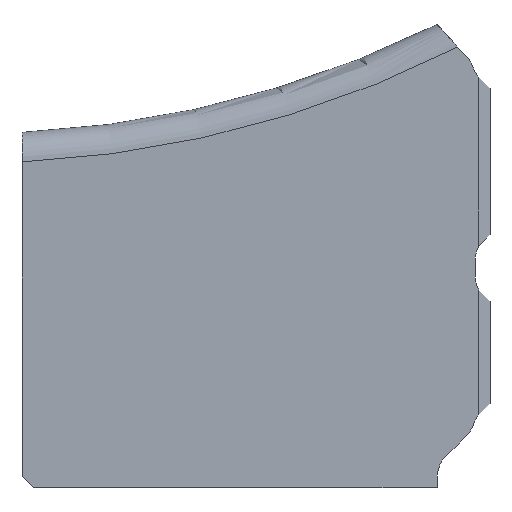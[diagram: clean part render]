
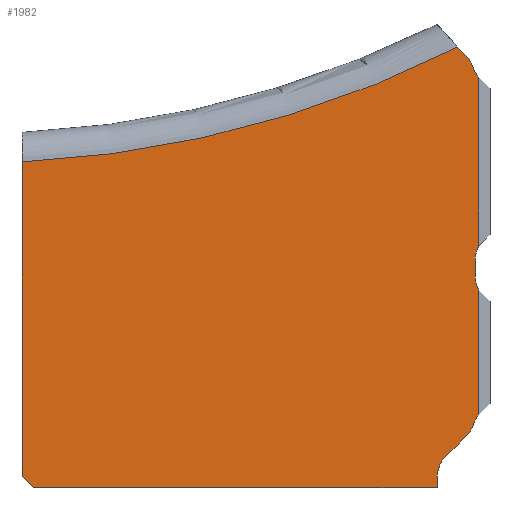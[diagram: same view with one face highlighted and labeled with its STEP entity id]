
A CAD part, front view. The second image highlights one B-rep face of the part: STEP entity #1982.
In plain terms, the highlighted planar face has unit normal (0, -1, 0).
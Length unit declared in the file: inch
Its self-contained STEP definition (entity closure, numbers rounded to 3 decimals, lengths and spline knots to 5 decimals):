
#145 = CIRCLE ( 'NONE', #2823, 0.3937 ) ;
#146 = CIRCLE ( 'NONE', #2832, 0.3937 ) ;
#149 = CIRCLE ( 'NONE', #2792, 0.3937 ) ;
#150 = CIRCLE ( 'NONE', #2861, 0.3937 ) ;
#164 = CIRCLE ( 'NONE', #2778, 14.52805 ) ;
#172 = CIRCLE ( 'NONE', #2789, 0.3937 ) ;
#173 = CIRCLE ( 'NONE', #2790, 0.3937 ) ;
#174 = CIRCLE ( 'NONE', #2833, 0.3937 ) ;
#375 = PLANE ( 'NONE',  #3064 ) ;
#376 = CARTESIAN_POINT ( 'NONE',  ( 0., 0., 0. ) ) ;
#379 = DIRECTION ( 'NONE',  ( 0., 1., 0. ) ) ;
#412 = DIRECTION ( 'NONE',  ( 0., 0., 1. ) ) ;
#1637 = CARTESIAN_POINT ( 'NONE',  ( 0., 0., 0. ) ) ;
#1642 = DIRECTION ( 'NONE',  ( 0., 0., -1. ) ) ;
#1646 = CARTESIAN_POINT ( 'NONE',  ( 5.66581, 0., 0.73541 ) ) ;
#1649 = DIRECTION ( 'NONE',  ( 0., -1., 0. ) ) ;
#1650 = LINE ( 'NONE', #1637, #2796 ) ;
#1663 = DIRECTION ( 'NONE',  ( 0., 1., 0. ) ) ;
#1670 = CARTESIAN_POINT ( 'NONE',  ( -0.70452, 0., 14.11678 ) ) ;
#1671 = DIRECTION ( 'NONE',  ( 0., 0., 1. ) ) ;
#1676 = LINE ( 'NONE', #1678, #2814 ) ;
#1677 = DIRECTION ( 'NONE',  ( 0.707, 0., 0.707 ) ) ;
#1678 = CARTESIAN_POINT ( 'NONE',  ( 5.00113, 0., -5.00113 ) ) ;
#1685 = DIRECTION ( 'NONE',  ( 0., 0., 1. ) ) ;
#1686 = CARTESIAN_POINT ( 'NONE',  ( 6.41166, 0., 0.9878 ) ) ;
#1687 = DIRECTION ( 'NONE',  ( 0., 0., 1. ) ) ;
#1688 = DIRECTION ( 'NONE',  ( 0., 1., 0. ) ) ;
#1690 = LINE ( 'NONE', #1691, #2801 ) ;
#1691 = CARTESIAN_POINT ( 'NONE',  ( 6.05951, 0., 0. ) ) ;
#1692 = DIRECTION ( 'NONE',  ( 0., 0., 1. ) ) ;
#1703 = LINE ( 'NONE', #1726, #2809 ) ;
#1711 = CARTESIAN_POINT ( 'NONE',  ( 6.10951, 0., 0. ) ) ;
#1718 = LINE ( 'NONE', #1711, #2817 ) ;
#1724 = DIRECTION ( 'NONE',  ( 0., 0., 1. ) ) ;
#1725 = DIRECTION ( 'NONE',  ( 0., 0., 1. ) ) ;
#1726 = CARTESIAN_POINT ( 'NONE',  ( 5.55226, 0., -4.75 ) ) ;
#1731 = DIRECTION ( 'NONE',  ( 0., 1., 0. ) ) ;
#1732 = CARTESIAN_POINT ( 'NONE',  ( 5.55226, 0., -4.75 ) ) ;
#1733 = DIRECTION ( 'NONE',  ( -1., 0., 0. ) ) ;
#1735 = LINE ( 'NONE', #1756, #2816 ) ;
#1739 = DIRECTION ( 'NONE',  ( 0.707, 0., -0.707 ) ) ;
#1741 = CARTESIAN_POINT ( 'NONE',  ( 6.45321, 0., -1.71415 ) ) ;
#1744 = LINE ( 'NONE', #1732, #2807 ) ;
#1753 = DIRECTION ( 'NONE',  ( 0., 0., 1. ) ) ;
#1756 = CARTESIAN_POINT ( 'NONE',  ( 0.15, 0., -4.75 ) ) ;
#1791 = LINE ( 'NONE', #1809, #2829 ) ;
#1792 = CARTESIAN_POINT ( 'NONE',  ( 6.10951, 0., 0. ) ) ;
#1800 = DIRECTION ( 'NONE',  ( -0.675, 0., 0.738 ) ) ;
#1802 = LINE ( 'NONE', #1792, #2831 ) ;
#1809 = CARTESIAN_POINT ( 'NONE',  ( 3.74048, 0., 3.42269 ) ) ;
#1818 = DIRECTION ( 'NONE',  ( 0., 0., 1. ) ) ;
#1854 = CARTESIAN_POINT ( 'NONE',  ( 6.41166, 0., -4.03208 ) ) ;
#1856 = DIRECTION ( 'NONE',  ( 0., 1., 0. ) ) ;
#1858 = CARTESIAN_POINT ( 'NONE',  ( 5.66581, 0., -3.77968 ) ) ;
#1859 = DIRECTION ( 'NONE',  ( 0., 0., 1. ) ) ;
#1982 = ADVANCED_FACE ( 'NONE', ( #3076 ), #375, .F. ) ;
#2295 = EDGE_CURVE ( 'NONE', #3464, #3466, #1650, .T. ) ;
#2296 = EDGE_CURVE ( 'NONE', #3444, #3505, #173, .T. ) ;
#2297 = EDGE_CURVE ( 'NONE', #3472, #3464, #164, .T. ) ;
#2299 = EDGE_CURVE ( 'NONE', #3498, #3481, #1690, .T. ) ;
#2303 = EDGE_CURVE ( 'NONE', #3455, #3444, #172, .T. ) ;
#2305 = EDGE_CURVE ( 'NONE', #3456, #3446, #1676, .T. ) ;
#2307 = EDGE_CURVE ( 'NONE', #3445, #3506, #1703, .T. ) ;
#2308 = EDGE_CURVE ( 'NONE', #3496, #3455, #1718, .T. ) ;
#2311 = EDGE_CURVE ( 'NONE', #3466, #3492, #1735, .T. ) ;
#2317 = EDGE_CURVE ( 'NONE', #3445, #3492, #1744, .T. ) ;
#2318 = EDGE_CURVE ( 'NONE', #3481, #3496, #149, .T. ) ;
#2326 = EDGE_CURVE ( 'NONE', #3505, #3472, #1791, .T. ) ;
#2327 = EDGE_CURVE ( 'NONE', #3478, #3484, #1802, .T. ) ;
#2338 = EDGE_CURVE ( 'NONE', #3502, #3478, #174, .T. ) ;
#2340 = EDGE_CURVE ( 'NONE', #3446, #3502, #145, .T. ) ;
#2356 = EDGE_CURVE ( 'NONE', #3484, #3498, #146, .T. ) ;
#2357 = EDGE_CURVE ( 'NONE', #3506, #3456, #150, .T. ) ;
#2778 = AXIS2_PLACEMENT_3D ( 'NONE', #1670, #1688, #1685 ) ;
#2789 = AXIS2_PLACEMENT_3D ( 'NONE', #1686, #1663, #1671 ) ;
#2790 = AXIS2_PLACEMENT_3D ( 'NONE', #1646, #1649, #1687 ) ;
#2792 = AXIS2_PLACEMENT_3D ( 'NONE', #1741, #1731, #1753 ) ;
#2796 = VECTOR ( 'NONE', #1642, 39.37008 ) ;
#2801 = VECTOR ( 'NONE', #1692, 39.37008 ) ;
#2807 = VECTOR ( 'NONE', #1733, 39.37008 ) ;
#2809 = VECTOR ( 'NONE', #1725, 39.37008 ) ;
#2814 = VECTOR ( 'NONE', #1677, 39.37008 ) ;
#2816 = VECTOR ( 'NONE', #1739, 39.37008 ) ;
#2817 = VECTOR ( 'NONE', #1724, 39.37008 ) ;
#2823 = AXIS2_PLACEMENT_3D ( 'NONE', #1858, #4702, #4010 ) ;
#2829 = VECTOR ( 'NONE', #1800, 39.37008 ) ;
#2831 = VECTOR ( 'NONE', #1818, 39.37008 ) ;
#2832 = AXIS2_PLACEMENT_3D ( 'NONE', #4058, #4080, #4078 ) ;
#2833 = AXIS2_PLACEMENT_3D ( 'NONE', #1854, #1856, #1859 ) ;
#2861 = AXIS2_PLACEMENT_3D ( 'NONE', #4064, #4086, #4059 ) ;
#2870 = EDGE_LOOP ( 'NONE', ( #3551, #3539, #3554, #3540, #3535, #3543, #3510, #3550, #3545, #3552, #3555, #3541, #3542, #3429, #3425, #3428, #3411 ) ) ;
#3064 = AXIS2_PLACEMENT_3D ( 'NONE', #376, #379, #412 ) ;
#3076 = FACE_OUTER_BOUND ( 'NONE', #2870, .T. ) ;
#3411 = ORIENTED_EDGE ( 'NONE', *, *, #2356, .T. ) ;
#3425 = ORIENTED_EDGE ( 'NONE', *, *, #2338, .T. ) ;
#3428 = ORIENTED_EDGE ( 'NONE', *, *, #2327, .T. ) ;
#3429 = ORIENTED_EDGE ( 'NONE', *, *, #2340, .T. ) ;
#3444 = VERTEX_POINT ( 'NONE', #4138 ) ;
#3445 = VERTEX_POINT ( 'NONE', #4146 ) ;
#3446 = VERTEX_POINT ( 'NONE', #4123 ) ;
#3455 = VERTEX_POINT ( 'NONE', #4125 ) ;
#3456 = VERTEX_POINT ( 'NONE', #4148 ) ;
#3464 = VERTEX_POINT ( 'NONE', #4181 ) ;
#3466 = VERTEX_POINT ( 'NONE', #4151 ) ;
#3472 = VERTEX_POINT ( 'NONE', #4179 ) ;
#3478 = VERTEX_POINT ( 'NONE', #4160 ) ;
#3481 = VERTEX_POINT ( 'NONE', #4176 ) ;
#3484 = VERTEX_POINT ( 'NONE', #4161 ) ;
#3492 = VERTEX_POINT ( 'NONE', #4156 ) ;
#3496 = VERTEX_POINT ( 'NONE', #4153 ) ;
#3498 = VERTEX_POINT ( 'NONE', #4175 ) ;
#3502 = VERTEX_POINT ( 'NONE', #4166 ) ;
#3505 = VERTEX_POINT ( 'NONE', #4169 ) ;
#3506 = VERTEX_POINT ( 'NONE', #4193 ) ;
#3510 = ORIENTED_EDGE ( 'NONE', *, *, #2297, .T. ) ;
#3535 = ORIENTED_EDGE ( 'NONE', *, *, #2296, .T. ) ;
#3539 = ORIENTED_EDGE ( 'NONE', *, *, #2318, .T. ) ;
#3540 = ORIENTED_EDGE ( 'NONE', *, *, #2303, .T. ) ;
#3541 = ORIENTED_EDGE ( 'NONE', *, *, #2357, .T. ) ;
#3542 = ORIENTED_EDGE ( 'NONE', *, *, #2305, .T. ) ;
#3543 = ORIENTED_EDGE ( 'NONE', *, *, #2326, .T. ) ;
#3545 = ORIENTED_EDGE ( 'NONE', *, *, #2311, .T. ) ;
#3550 = ORIENTED_EDGE ( 'NONE', *, *, #2295, .T. ) ;
#3551 = ORIENTED_EDGE ( 'NONE', *, *, #2299, .T. ) ;
#3552 = ORIENTED_EDGE ( 'NONE', *, *, #2317, .F. ) ;
#3554 = ORIENTED_EDGE ( 'NONE', *, *, #2308, .T. ) ;
#3555 = ORIENTED_EDGE ( 'NONE', *, *, #2307, .T. ) ;
#4010 = DIRECTION ( 'NONE',  ( 0., 0., 1. ) ) ;
#4058 = CARTESIAN_POINT ( 'NONE',  ( 6.45321, 0., -1.91784 ) ) ;
#4059 = DIRECTION ( 'NONE',  ( 0., 0., 1. ) ) ;
#4064 = CARTESIAN_POINT ( 'NONE',  ( 5.94596, 0., -4.61308 ) ) ;
#4078 = DIRECTION ( 'NONE',  ( 0., 0., 1. ) ) ;
#4080 = DIRECTION ( 'NONE',  ( 0., 1., 0. ) ) ;
#4086 = DIRECTION ( 'NONE',  ( 0., 1., 0. ) ) ;
#4123 = CARTESIAN_POINT ( 'NONE',  ( 5.9442, 0., -4.05807 ) ) ;
#4125 = CARTESIAN_POINT ( 'NONE',  ( 6.10951, 0., 0.73541 ) ) ;
#4138 = CARTESIAN_POINT ( 'NONE',  ( 6.03873, 0., 0.86161 ) ) ;
#4146 = CARTESIAN_POINT ( 'NONE',  ( 5.55226, 0., -4.75 ) ) ;
#4148 = CARTESIAN_POINT ( 'NONE',  ( 5.66758, 0., -4.33469 ) ) ;
#4151 = CARTESIAN_POINT ( 'NONE',  ( 0., 0., -4.6 ) ) ;
#4153 = CARTESIAN_POINT ( 'NONE',  ( 6.10951, 0., -1.52214 ) ) ;
#4156 = CARTESIAN_POINT ( 'NONE',  ( 0.15, 0., -4.75 ) ) ;
#4160 = CARTESIAN_POINT ( 'NONE',  ( 6.10951, 0., -3.77968 ) ) ;
#4161 = CARTESIAN_POINT ( 'NONE',  ( 6.10951, 0., -2.10985 ) ) ;
#4166 = CARTESIAN_POINT ( 'NONE',  ( 6.03873, 0., -3.90588 ) ) ;
#4169 = CARTESIAN_POINT ( 'NONE',  ( 5.95626, 0., 1.00118 ) ) ;
#4175 = CARTESIAN_POINT ( 'NONE',  ( 6.05951, 0., -1.91784 ) ) ;
#4176 = CARTESIAN_POINT ( 'NONE',  ( 6.05951, 0., -1.71415 ) ) ;
#4179 = CARTESIAN_POINT ( 'NONE',  ( 5.82869, 0., 1.14059 ) ) ;
#4181 = CARTESIAN_POINT ( 'NONE',  ( 0., 0., -0.39418 ) ) ;
#4193 = CARTESIAN_POINT ( 'NONE',  ( 5.55226, 0., -4.61308 ) ) ;
#4702 = DIRECTION ( 'NONE',  ( 0., -1., 0. ) ) ;
